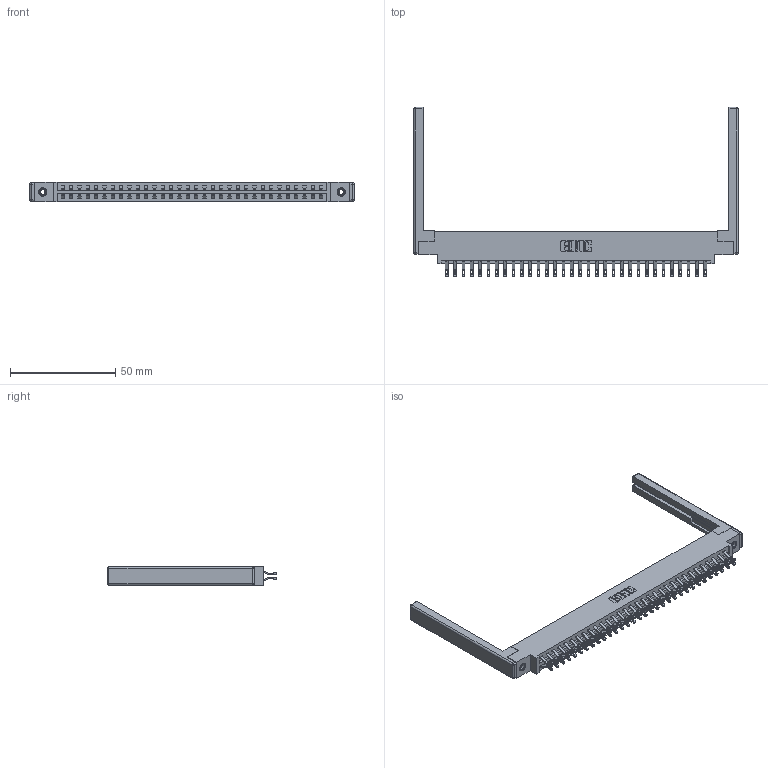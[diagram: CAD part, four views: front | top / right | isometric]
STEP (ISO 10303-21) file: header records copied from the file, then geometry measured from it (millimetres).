
FILE_DESCRIPTION (( 'STEP AP203' ), '1' );
FILE_NAME ('337-064-555-868.STEP', '2019-10-12T00:06:56', ( '' ), ( '' ), 'SwSTEP 2.0', 'SolidWorks 2016', '' );
FILE_SCHEMA (( 'CONFIG_CONTROL_DESIGN' ));
Length unit declared in the file: inch
Products named in the file (5): 337 Part_0.170 Offset - 0.156 Dia-TI; 307-220-068; 337-064-555-868; 345-250-001_345-250-001-102; 345-292-001_555 Tail
Assembly tree (69 placements, depth 2):
  337-064-555-868
    337 Part_0.170 Offset - 0.156 Dia-TI
    345-292-001_555 Tail  x64
    345-250-001_345-250-001-102  x2
    307-220-068  x2
Bounding box: 154.23 x 80.52 x 9.4 mm (x, y, z)
Volume: 20573.7 mm3; surface area: 23046.2 mm2
Topology: 69 solids, 69 shells, 4112 faces, 12809 edges, 8518 vertices
Faces by surface type: plane 2466, cylinder 1622, cone 12, sphere 8, torus 4
Entity records: 29322 total; most frequent: CARTESIAN_POINT 4949, ORIENTED_EDGE 4844, DIRECTION 4268, EDGE_CURVE 2422, LINE 2224, VECTOR 2224, VERTEX_POINT 1606, AXIS2_PLACEMENT_3D 1022
